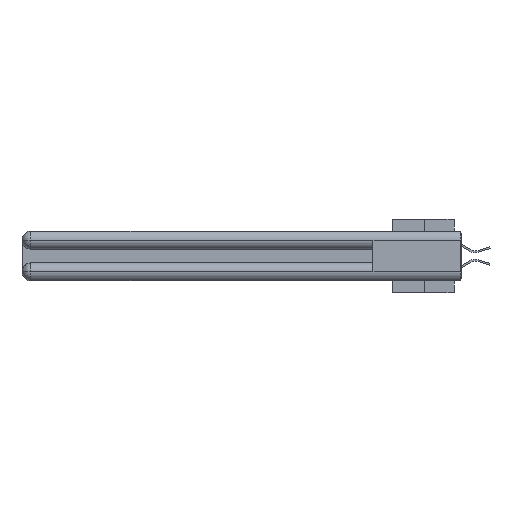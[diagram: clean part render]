
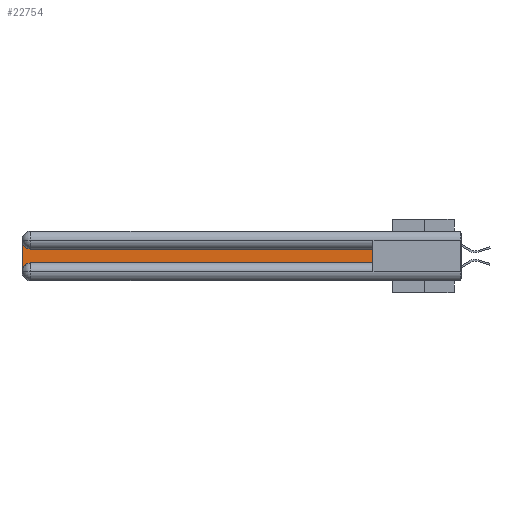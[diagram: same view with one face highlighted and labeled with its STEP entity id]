
A CAD part, left-side view. The second image highlights one B-rep face of the part: STEP entity #22754.
In plain terms, the highlighted planar face has unit normal (-1, 0, 0).
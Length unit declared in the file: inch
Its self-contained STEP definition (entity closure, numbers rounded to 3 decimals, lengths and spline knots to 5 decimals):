
#23 = EDGE_CURVE ( 'NONE', #12480, #9511, #30770, .T. ) ;
#1271 = ORIENTED_EDGE ( 'NONE', *, *, #27801, .T. ) ;
#1439 = CARTESIAN_POINT ( 'NONE',  ( 0.075, 0.6, -0.2175 ) ) ;
#2351 = DIRECTION ( 'NONE',  ( 0., 0., -1. ) ) ;
#2844 = CARTESIAN_POINT ( 'NONE',  ( 0.075, 2.94, -0.1225 ) ) ;
#3395 = CARTESIAN_POINT ( 'NONE',  ( 0.075, 3., -0.0625 ) ) ;
#4046 = LINE ( 'NONE', #8682, #10951 ) ;
#4918 = LINE ( 'NONE', #28997, #21344 ) ;
#5104 = DIRECTION ( 'NONE',  ( 0., 0., -1. ) ) ;
#5292 = ORIENTED_EDGE ( 'NONE', *, *, #22427, .T. ) ;
#5445 = AXIS2_PLACEMENT_3D ( 'NONE', #14318, #28904, #26507 ) ;
#6432 = CARTESIAN_POINT ( 'NONE',  ( 0.075, 2.94, -0.0625 ) ) ;
#6877 = DIRECTION ( 'NONE',  ( 1., 0., 0. ) ) ;
#8330 = VERTEX_POINT ( 'NONE', #28344 ) ;
#8626 = ORIENTED_EDGE ( 'NONE', *, *, #21203, .T. ) ;
#8682 = CARTESIAN_POINT ( 'NONE',  ( 0.075, 0.6, -0.2175 ) ) ;
#9424 = CARTESIAN_POINT ( 'NONE',  ( 0.075, 3., -0.1225 ) ) ;
#9511 = VERTEX_POINT ( 'NONE', #29788 ) ;
#10447 = CARTESIAN_POINT ( 'NONE',  ( 0.075, 3., -0.2775 ) ) ;
#10951 = VECTOR ( 'NONE', #23597, 39.37008 ) ;
#12480 = VERTEX_POINT ( 'NONE', #14593 ) ;
#13390 = VECTOR ( 'NONE', #18430, 39.37008 ) ;
#13481 = EDGE_LOOP ( 'NONE', ( #5292, #8626, #21217, #29402, #23847, #1271 ) ) ;
#13631 = DIRECTION ( 'NONE',  ( 0., 0., -1. ) ) ;
#14140 = CIRCLE ( 'NONE', #5445, 0.06 ) ;
#14318 = CARTESIAN_POINT ( 'NONE',  ( 0.075, 2.94, -0.2775 ) ) ;
#14593 = CARTESIAN_POINT ( 'NONE',  ( 0.075, 2.94, -0.2175 ) ) ;
#15915 = VECTOR ( 'NONE', #25035, 39.37008 ) ;
#16423 = AXIS2_PLACEMENT_3D ( 'NONE', #9424, #6877, #5104 ) ;
#16656 = EDGE_CURVE ( 'NONE', #27697, #12480, #14140, .T. ) ;
#17374 = AXIS2_PLACEMENT_3D ( 'NONE', #6432, #25829, #13631 ) ;
#18430 = DIRECTION ( 'NONE',  ( 0., -1., 0. ) ) ;
#18646 = EDGE_CURVE ( 'NONE', #30710, #27697, #4918, .T. ) ;
#21203 = EDGE_CURVE ( 'NONE', #29738, #30710, #26088, .T. ) ;
#21217 = ORIENTED_EDGE ( 'NONE', *, *, #18646, .T. ) ;
#21344 = VECTOR ( 'NONE', #2351, 39.37008 ) ;
#22427 = EDGE_CURVE ( 'NONE', #8330, #29738, #27284, .T. ) ;
#22754 = ADVANCED_FACE ( 'NONE', ( #28833 ), #28985, .F. ) ;
#23597 = DIRECTION ( 'NONE',  ( 0., 0., 1. ) ) ;
#23847 = ORIENTED_EDGE ( 'NONE', *, *, #23, .T. ) ;
#25035 = DIRECTION ( 'NONE',  ( 0., 1., 0. ) ) ;
#25829 = DIRECTION ( 'NONE',  ( 1., 0., 0. ) ) ;
#26088 = CIRCLE ( 'NONE', #17374, 0.06 ) ;
#26507 = DIRECTION ( 'NONE',  ( 0., 0., -1. ) ) ;
#27284 = LINE ( 'NONE', #29685, #15915 ) ;
#27697 = VERTEX_POINT ( 'NONE', #10447 ) ;
#27801 = EDGE_CURVE ( 'NONE', #9511, #8330, #4046, .T. ) ;
#28344 = CARTESIAN_POINT ( 'NONE',  ( 0.075, 0.6, -0.1225 ) ) ;
#28833 = FACE_OUTER_BOUND ( 'NONE', #13481, .T. ) ;
#28904 = DIRECTION ( 'NONE',  ( 1., 0., 0. ) ) ;
#28985 = PLANE ( 'NONE',  #16423 ) ;
#28997 = CARTESIAN_POINT ( 'NONE',  ( 0.075, 3., -0.2175 ) ) ;
#29402 = ORIENTED_EDGE ( 'NONE', *, *, #16656, .T. ) ;
#29685 = CARTESIAN_POINT ( 'NONE',  ( 0.075, 0.6, -0.1225 ) ) ;
#29738 = VERTEX_POINT ( 'NONE', #2844 ) ;
#29788 = CARTESIAN_POINT ( 'NONE',  ( 0.075, 0.6, -0.2175 ) ) ;
#30710 = VERTEX_POINT ( 'NONE', #3395 ) ;
#30770 = LINE ( 'NONE', #1439, #13390 ) ;
